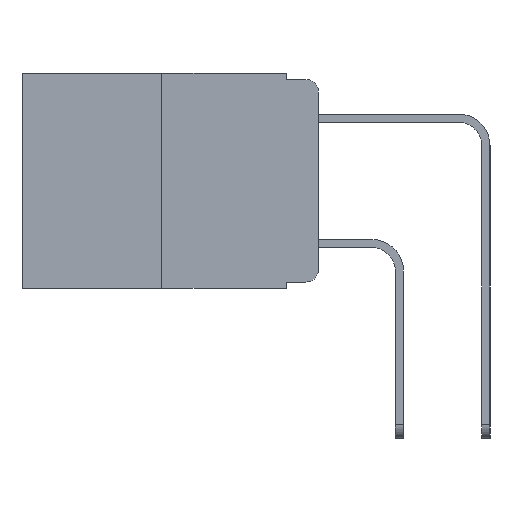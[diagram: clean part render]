
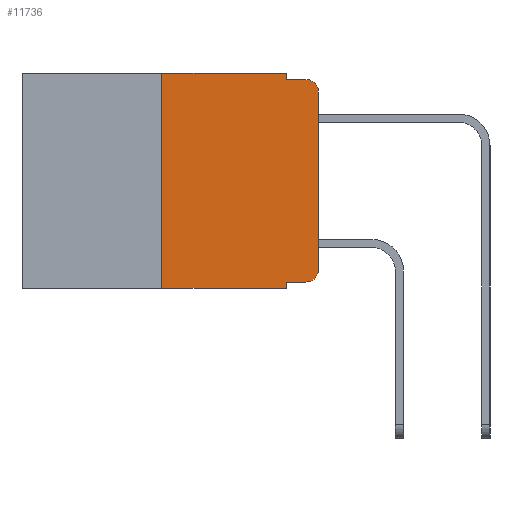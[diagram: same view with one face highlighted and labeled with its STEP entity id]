
A CAD part, left-side view. The second image highlights one B-rep face of the part: STEP entity #11736.
In plain terms, the highlighted planar face has unit normal (-1, 0, 0).
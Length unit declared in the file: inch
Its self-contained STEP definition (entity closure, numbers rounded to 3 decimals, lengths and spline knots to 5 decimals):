
#28 = DIRECTION ( 'NONE',  ( 0., 0., -1. ) ) ;
#284 = CARTESIAN_POINT ( 'NONE',  ( 0., 0.02, -0.333 ) ) ;
#317 = CARTESIAN_POINT ( 'NONE',  ( 0., 0.051, -0.333 ) ) ;
#372 = DIRECTION ( 'NONE',  ( 1., 0., 0. ) ) ;
#437 = DIRECTION ( 'NONE',  ( 0., -1., 0. ) ) ;
#950 = VECTOR ( 'NONE', #8408, 39.37008 ) ;
#1069 = CARTESIAN_POINT ( 'NONE',  ( 0., 0.473, -0.343 ) ) ;
#1233 = LINE ( 'NONE', #4343, #8774 ) ;
#1576 = CARTESIAN_POINT ( 'NONE',  ( 0., 0.25, 0. ) ) ;
#2088 = DIRECTION ( 'NONE',  ( 0., -1., 0. ) ) ;
#3115 = CARTESIAN_POINT ( 'NONE',  ( 0., 0.473, 0. ) ) ;
#3309 = LINE ( 'NONE', #7441, #950 ) ;
#3629 = ORIENTED_EDGE ( 'NONE', *, *, #9185, .T. ) ;
#3647 = ORIENTED_EDGE ( 'NONE', *, *, #7734, .F. ) ;
#3695 = CARTESIAN_POINT ( 'NONE',  ( 0., 0.02, -0.313 ) ) ;
#3916 = LINE ( 'NONE', #1069, #6201 ) ;
#4062 = VERTEX_POINT ( 'NONE', #9078 ) ;
#4256 = LINE ( 'NONE', #5148, #9123 ) ;
#4316 = VERTEX_POINT ( 'NONE', #6215 ) ;
#4343 = CARTESIAN_POINT ( 'NONE',  ( 0., 0.051, -0.01 ) ) ;
#4369 = FACE_OUTER_BOUND ( 'NONE', #8006, .T. ) ;
#4456 = AXIS2_PLACEMENT_3D ( 'NONE', #6295, #372, #7289 ) ;
#4511 = VERTEX_POINT ( 'NONE', #8863 ) ;
#4663 = DIRECTION ( 'NONE',  ( 0., 0., -1. ) ) ;
#4914 = LINE ( 'NONE', #3115, #12290 ) ;
#5125 = VERTEX_POINT ( 'NONE', #9293 ) ;
#5148 = CARTESIAN_POINT ( 'NONE',  ( 0., 0., 0. ) ) ;
#5159 = LINE ( 'NONE', #1576, #7165 ) ;
#5408 = EDGE_CURVE ( 'NONE', #5950, #11895, #9517, .T. ) ;
#5478 = ORIENTED_EDGE ( 'NONE', *, *, #5699, .F. ) ;
#5484 = AXIS2_PLACEMENT_3D ( 'NONE', #11755, #5963, #28 ) ;
#5567 = CARTESIAN_POINT ( 'NONE',  ( 0., 0.051, -0.343 ) ) ;
#5699 = EDGE_CURVE ( 'NONE', #9656, #5125, #1233, .T. ) ;
#5950 = VERTEX_POINT ( 'NONE', #8690 ) ;
#5963 = DIRECTION ( 'NONE',  ( -1., 0., 0. ) ) ;
#6201 = VECTOR ( 'NONE', #8930, 39.37008 ) ;
#6215 = CARTESIAN_POINT ( 'NONE',  ( 0., 0.25, -0.343 ) ) ;
#6295 = CARTESIAN_POINT ( 'NONE',  ( 0., 0.473, 0. ) ) ;
#6385 = EDGE_CURVE ( 'NONE', #11709, #7771, #7864, .T. ) ;
#6386 = ORIENTED_EDGE ( 'NONE', *, *, #11551, .T. ) ;
#6435 = LINE ( 'NONE', #317, #9006 ) ;
#6540 = DIRECTION ( 'NONE',  ( 0., 0., 1. ) ) ;
#6713 = ORIENTED_EDGE ( 'NONE', *, *, #11204, .F. ) ;
#6836 = ORIENTED_EDGE ( 'NONE', *, *, #10257, .T. ) ;
#6891 = DIRECTION ( 'NONE',  ( 0., 0., -1. ) ) ;
#7101 = CARTESIAN_POINT ( 'NONE',  ( 0., 0., -0.313 ) ) ;
#7165 = VECTOR ( 'NONE', #6540, 39.37008 ) ;
#7289 = DIRECTION ( 'NONE',  ( 0., 0., -1. ) ) ;
#7441 = CARTESIAN_POINT ( 'NONE',  ( 0., 0.051, 0. ) ) ;
#7734 = EDGE_CURVE ( 'NONE', #10052, #4062, #4914, .T. ) ;
#7771 = VERTEX_POINT ( 'NONE', #7101 ) ;
#7864 = CIRCLE ( 'NONE', #8329, 0.02 ) ;
#8006 = EDGE_LOOP ( 'NONE', ( #6836, #12498, #5478, #6713, #3647, #11975, #6386, #12368, #3629, #12246 ) ) ;
#8104 = DIRECTION ( 'NONE',  ( 0., 0., 1. ) ) ;
#8207 = DIRECTION ( 'NONE',  ( 0., -1., 0. ) ) ;
#8329 = AXIS2_PLACEMENT_3D ( 'NONE', #3695, #10482, #4663 ) ;
#8332 = EDGE_CURVE ( 'NONE', #4511, #5125, #8574, .T. ) ;
#8408 = DIRECTION ( 'NONE',  ( 0., 0., -1. ) ) ;
#8574 = CIRCLE ( 'NONE', #5484, 0.02 ) ;
#8690 = CARTESIAN_POINT ( 'NONE',  ( 0., 0.051, -0.333 ) ) ;
#8774 = VECTOR ( 'NONE', #437, 39.37008 ) ;
#8863 = CARTESIAN_POINT ( 'NONE',  ( 0., 0., -0.03 ) ) ;
#8930 = DIRECTION ( 'NONE',  ( 0., -1., 0. ) ) ;
#9006 = VECTOR ( 'NONE', #8207, 39.37008 ) ;
#9078 = CARTESIAN_POINT ( 'NONE',  ( 0., 0.051, 0. ) ) ;
#9123 = VECTOR ( 'NONE', #8104, 39.37008 ) ;
#9164 = CARTESIAN_POINT ( 'NONE',  ( 0., 0.051, -0.01 ) ) ;
#9185 = EDGE_CURVE ( 'NONE', #5950, #11709, #6435, .T. ) ;
#9293 = CARTESIAN_POINT ( 'NONE',  ( 0., 0.02, -0.01 ) ) ;
#9517 = LINE ( 'NONE', #12549, #11774 ) ;
#9656 = VERTEX_POINT ( 'NONE', #9164 ) ;
#10052 = VERTEX_POINT ( 'NONE', #10705 ) ;
#10137 = PLANE ( 'NONE',  #4456 ) ;
#10257 = EDGE_CURVE ( 'NONE', #7771, #4511, #4256, .T. ) ;
#10482 = DIRECTION ( 'NONE',  ( -1., 0., 0. ) ) ;
#10594 = EDGE_CURVE ( 'NONE', #4316, #10052, #5159, .T. ) ;
#10705 = CARTESIAN_POINT ( 'NONE',  ( 0., 0.25, 0. ) ) ;
#11204 = EDGE_CURVE ( 'NONE', #4062, #9656, #3309, .T. ) ;
#11551 = EDGE_CURVE ( 'NONE', #4316, #11895, #3916, .T. ) ;
#11709 = VERTEX_POINT ( 'NONE', #284 ) ;
#11736 = ADVANCED_FACE ( 'NONE', ( #4369 ), #10137, .F. ) ;
#11755 = CARTESIAN_POINT ( 'NONE',  ( 0., 0.02, -0.03 ) ) ;
#11774 = VECTOR ( 'NONE', #6891, 39.37008 ) ;
#11895 = VERTEX_POINT ( 'NONE', #5567 ) ;
#11975 = ORIENTED_EDGE ( 'NONE', *, *, #10594, .F. ) ;
#12246 = ORIENTED_EDGE ( 'NONE', *, *, #6385, .T. ) ;
#12290 = VECTOR ( 'NONE', #2088, 39.37008 ) ;
#12368 = ORIENTED_EDGE ( 'NONE', *, *, #5408, .F. ) ;
#12498 = ORIENTED_EDGE ( 'NONE', *, *, #8332, .T. ) ;
#12549 = CARTESIAN_POINT ( 'NONE',  ( 0., 0.051, 0. ) ) ;
